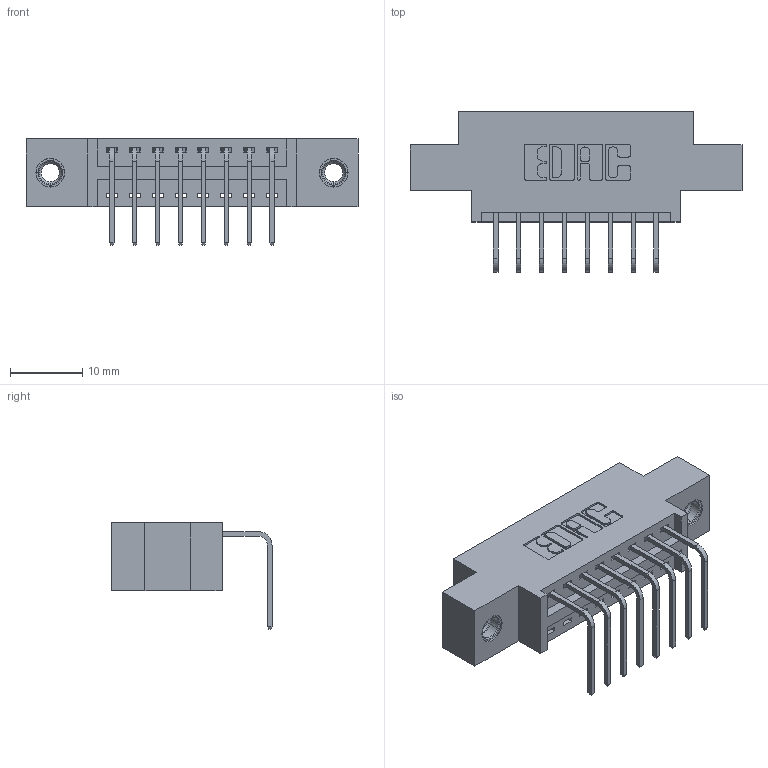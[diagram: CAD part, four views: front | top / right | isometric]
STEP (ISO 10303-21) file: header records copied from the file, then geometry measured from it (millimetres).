
FILE_DESCRIPTION (( 'STEP AP203' ), '1' );
FILE_NAME ('346-008-558-607.STEP', '2022-05-04T21:35:34', ( '' ), ( '' ), 'SwSTEP 2.0', 'SolidWorks 2020', '' );
FILE_SCHEMA (( 'CONFIG_CONTROL_DESIGN' ));
Length unit declared in the file: inch
Products named in the file (4): 345-250-001_345-250-005-103; 346 Part_0.170 Offset - 0.156 Dia-TI; 346-008-558-607; 345-292-001_558 Tail - 2
Assembly tree (11 placements, depth 2):
  346-008-558-607
    346 Part_0.170 Offset - 0.156 Dia-TI
    345-292-001_558 Tail - 2  x8
    345-250-001_345-250-005-103  x2
Bounding box: 45.97 x 22.16 x 14.73 mm (x, y, z)
Volume: 4025 mm3; surface area: 5017.8 mm2
Topology: 11 solids, 11 shells, 666 faces, 1933 edges, 1270 vertices
Faces by surface type: plane 448, cylinder 202, cone 12, torus 4
Entity records: 10944 total; most frequent: CARTESIAN_POINT 1871, ORIENTED_EDGE 1806, DIRECTION 1717, EDGE_CURVE 903, LINE 719, VECTOR 719, VERTEX_POINT 596, AXIS2_PLACEMENT_3D 499
